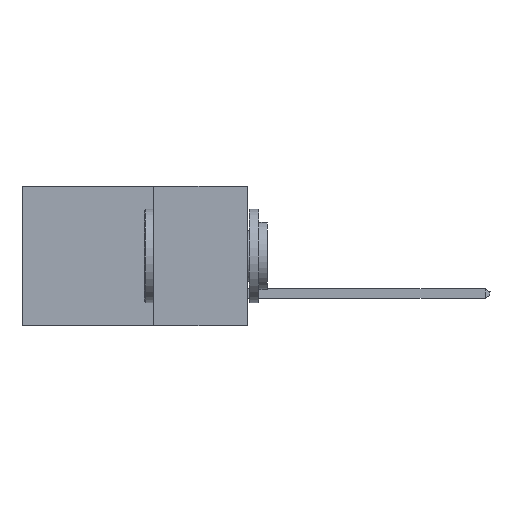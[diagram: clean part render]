
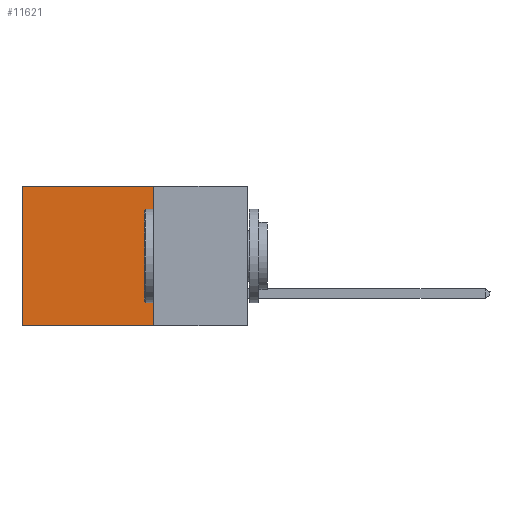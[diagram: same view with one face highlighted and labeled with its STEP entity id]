
A CAD part, left-side view. The second image highlights one B-rep face of the part: STEP entity #11621.
In plain terms, the highlighted planar face has unit normal (-1, 0, 0).
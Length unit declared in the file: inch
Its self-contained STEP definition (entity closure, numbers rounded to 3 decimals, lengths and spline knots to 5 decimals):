
#66 = VERTEX_POINT ( 'NONE', #12499 ) ;
#301 = CARTESIAN_POINT ( 'NONE',  ( 0.2615, 0.6, -0.37 ) ) ;
#565 = CARTESIAN_POINT ( 'NONE',  ( 0.2615, 0.25, -0.37 ) ) ;
#702 = VECTOR ( 'NONE', #3595, 39.37008 ) ;
#818 = AXIS2_PLACEMENT_3D ( 'NONE', #7889, #8092, #8814 ) ;
#871 = PLANE ( 'NONE',  #818 ) ;
#1849 = DIRECTION ( 'NONE',  ( 0., 0., -1. ) ) ;
#1860 = FACE_OUTER_BOUND ( 'NONE', #3832, .T. ) ;
#2118 = EDGE_CURVE ( 'NONE', #6106, #12924, #8281, .T. ) ;
#2152 = CARTESIAN_POINT ( 'NONE',  ( 0.2615, 0.25, 0. ) ) ;
#2629 = CARTESIAN_POINT ( 'NONE',  ( 0.2615, 0.25, 0. ) ) ;
#3071 = ORIENTED_EDGE ( 'NONE', *, *, #7232, .F. ) ;
#3188 = DIRECTION ( 'NONE',  ( 0., 1., 0. ) ) ;
#3595 = DIRECTION ( 'NONE',  ( 0., 0., -1. ) ) ;
#3832 = EDGE_LOOP ( 'NONE', ( #10476, #3071, #8217, #4610 ) ) ;
#3958 = CARTESIAN_POINT ( 'NONE',  ( 0.2615, 0.6, -0.37 ) ) ;
#3985 = LINE ( 'NONE', #2152, #13348 ) ;
#4610 = ORIENTED_EDGE ( 'NONE', *, *, #10772, .T. ) ;
#5019 = VECTOR ( 'NONE', #3188, 39.37008 ) ;
#5129 = DIRECTION ( 'NONE',  ( 0., 1., 0. ) ) ;
#6106 = VERTEX_POINT ( 'NONE', #8243 ) ;
#6805 = EDGE_CURVE ( 'NONE', #13332, #66, #9810, .T. ) ;
#7232 = EDGE_CURVE ( 'NONE', #66, #12924, #10496, .T. ) ;
#7889 = CARTESIAN_POINT ( 'NONE',  ( 0.2615, 0.25, -0.37 ) ) ;
#8092 = DIRECTION ( 'NONE',  ( 1., 0., 0. ) ) ;
#8217 = ORIENTED_EDGE ( 'NONE', *, *, #6805, .F. ) ;
#8243 = CARTESIAN_POINT ( 'NONE',  ( 0.2615, 0.6, 0. ) ) ;
#8281 = LINE ( 'NONE', #3958, #11902 ) ;
#8582 = CARTESIAN_POINT ( 'NONE',  ( 0.2615, 0.25, -0.37 ) ) ;
#8814 = DIRECTION ( 'NONE',  ( 0., 0., -1. ) ) ;
#9810 = LINE ( 'NONE', #565, #702 ) ;
#10476 = ORIENTED_EDGE ( 'NONE', *, *, #2118, .T. ) ;
#10496 = LINE ( 'NONE', #8582, #5019 ) ;
#10772 = EDGE_CURVE ( 'NONE', #13332, #6106, #3985, .T. ) ;
#11621 = ADVANCED_FACE ( 'NONE', ( #1860 ), #871, .F. ) ;
#11902 = VECTOR ( 'NONE', #1849, 39.37008 ) ;
#12499 = CARTESIAN_POINT ( 'NONE',  ( 0.2615, 0.25, -0.37 ) ) ;
#12924 = VERTEX_POINT ( 'NONE', #301 ) ;
#13332 = VERTEX_POINT ( 'NONE', #2629 ) ;
#13348 = VECTOR ( 'NONE', #5129, 39.37008 ) ;
